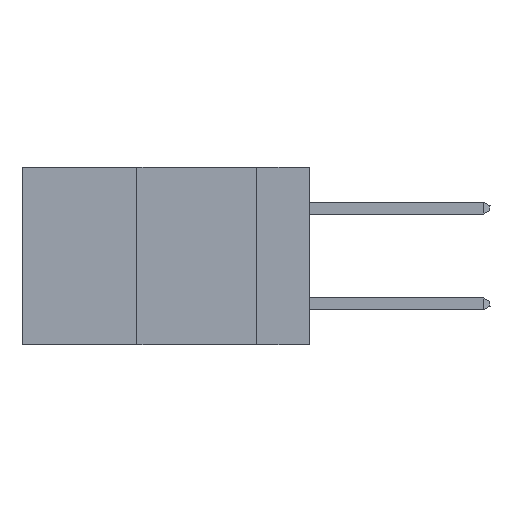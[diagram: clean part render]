
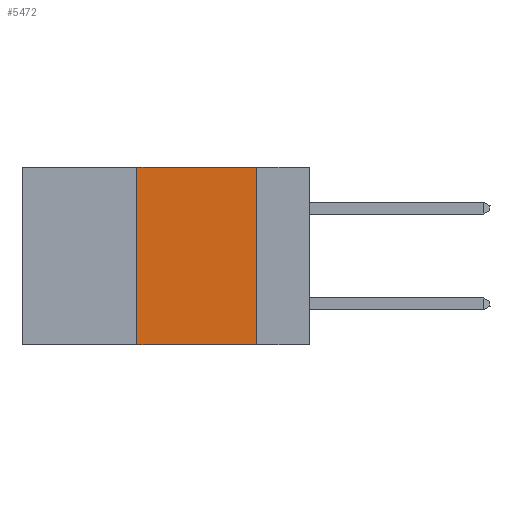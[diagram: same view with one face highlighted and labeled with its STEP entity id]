
A CAD part, left-side view. The second image highlights one B-rep face of the part: STEP entity #5472.
In plain terms, the highlighted planar face has unit normal (-1, 0, 0).
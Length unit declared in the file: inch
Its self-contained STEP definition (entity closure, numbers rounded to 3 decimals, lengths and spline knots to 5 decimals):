
#768 = EDGE_LOOP ( 'NONE', ( #873, #17122, #20648, #21043 ) ) ;
#812 = LINE ( 'NONE', #4399, #7288 ) ;
#870 = DIRECTION ( 'NONE',  ( 0., 0., -1. ) ) ;
#873 = ORIENTED_EDGE ( 'NONE', *, *, #17114, .F. ) ;
#2182 = VERTEX_POINT ( 'NONE', #2365 ) ;
#2365 = CARTESIAN_POINT ( 'NONE',  ( 0., 0.36, -0.37 ) ) ;
#2582 = LINE ( 'NONE', #6796, #12434 ) ;
#2854 = CARTESIAN_POINT ( 'NONE',  ( 0., 0.36, 0. ) ) ;
#4388 = CARTESIAN_POINT ( 'NONE',  ( 0., 0.11, 0. ) ) ;
#4399 = CARTESIAN_POINT ( 'NONE',  ( 0., 0.6, 0. ) ) ;
#5283 = AXIS2_PLACEMENT_3D ( 'NONE', #19377, #23078, #870 ) ;
#5472 = ADVANCED_FACE ( 'NONE', ( #8408 ), #13405, .F. ) ;
#6796 = CARTESIAN_POINT ( 'NONE',  ( 0., 0.36, 0. ) ) ;
#7133 = DIRECTION ( 'NONE',  ( 0., 0., 1. ) ) ;
#7288 = VECTOR ( 'NONE', #22906, 39.37008 ) ;
#8129 = CARTESIAN_POINT ( 'NONE',  ( 0., 0.11, -0.37 ) ) ;
#8408 = FACE_OUTER_BOUND ( 'NONE', #768, .T. ) ;
#11052 = VECTOR ( 'NONE', #18010, 39.37008 ) ;
#12139 = EDGE_CURVE ( 'NONE', #2182, #15593, #2582, .T. ) ;
#12344 = CARTESIAN_POINT ( 'NONE',  ( 0., 0.6, -0.37 ) ) ;
#12434 = VECTOR ( 'NONE', #7133, 39.37008 ) ;
#13405 = PLANE ( 'NONE',  #5283 ) ;
#13530 = LINE ( 'NONE', #4388, #19967 ) ;
#14981 = DIRECTION ( 'NONE',  ( 0., 0., -1. ) ) ;
#15473 = EDGE_CURVE ( 'NONE', #2182, #21643, #21475, .T. ) ;
#15593 = VERTEX_POINT ( 'NONE', #2854 ) ;
#15910 = CARTESIAN_POINT ( 'NONE',  ( 0., 0.11, 0. ) ) ;
#16781 = EDGE_CURVE ( 'NONE', #15593, #23302, #812, .T. ) ;
#17114 = EDGE_CURVE ( 'NONE', #23302, #21643, #13530, .T. ) ;
#17122 = ORIENTED_EDGE ( 'NONE', *, *, #16781, .F. ) ;
#18010 = DIRECTION ( 'NONE',  ( 0., -1., 0. ) ) ;
#19377 = CARTESIAN_POINT ( 'NONE',  ( 0., 0.6, 0. ) ) ;
#19967 = VECTOR ( 'NONE', #14981, 39.37008 ) ;
#20648 = ORIENTED_EDGE ( 'NONE', *, *, #12139, .F. ) ;
#21043 = ORIENTED_EDGE ( 'NONE', *, *, #15473, .T. ) ;
#21475 = LINE ( 'NONE', #12344, #11052 ) ;
#21643 = VERTEX_POINT ( 'NONE', #8129 ) ;
#22906 = DIRECTION ( 'NONE',  ( 0., -1., 0. ) ) ;
#23078 = DIRECTION ( 'NONE',  ( 1., 0., 0. ) ) ;
#23302 = VERTEX_POINT ( 'NONE', #15910 ) ;
